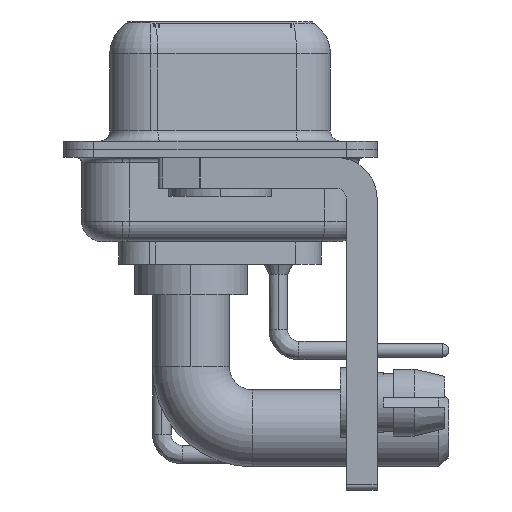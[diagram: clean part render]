
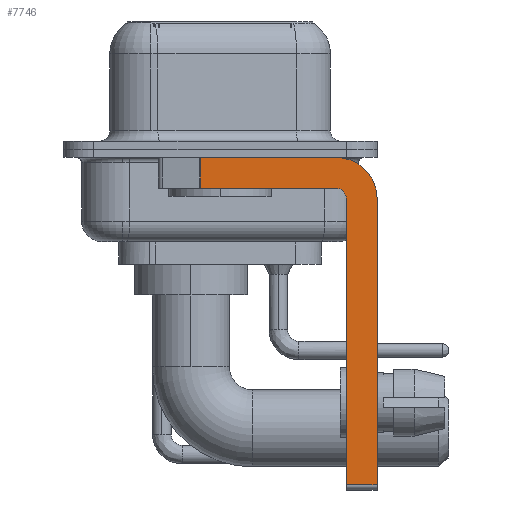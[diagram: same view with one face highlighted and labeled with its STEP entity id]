
A CAD part, left-side view. The second image highlights one B-rep face of the part: STEP entity #7746.
In plain terms, the highlighted planar face has unit normal (-1, 0, 0).
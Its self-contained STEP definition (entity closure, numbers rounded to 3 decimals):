
#274 = ORIENTED_EDGE ( 'NONE', *, *, #30336, .F. ) ;
#1246 = CARTESIAN_POINT ( 'NONE',  ( -2.9, -5.65, -16.35 ) ) ;
#1371 = AXIS2_PLACEMENT_3D ( 'NONE', #30924, #18235, #26679 ) ;
#1701 = CARTESIAN_POINT ( 'NONE',  ( -2.9, 0.978, -1.9 ) ) ;
#1873 = LINE ( 'NONE', #1701, #7406 ) ;
#1939 = DIRECTION ( 'NONE',  ( 0., 0., 1. ) ) ;
#2439 = EDGE_CURVE ( 'NONE', #2529, #18310, #12420, .T. ) ;
#2529 = VERTEX_POINT ( 'NONE', #21902 ) ;
#2671 = CIRCLE ( 'NONE', #26394, 2. ) ;
#3564 = CARTESIAN_POINT ( 'NONE',  ( -2.9, -5.65, -0.4 ) ) ;
#4434 = DIRECTION ( 'NONE',  ( -1., 0., 0. ) ) ;
#4453 = VERTEX_POINT ( 'NONE', #32727 ) ;
#5607 = VECTOR ( 'NONE', #20358, 1000. ) ;
#6105 = CARTESIAN_POINT ( 'NONE',  ( -2.9, 0.978, -1.9 ) ) ;
#6236 = CARTESIAN_POINT ( 'NONE',  ( -2.9, -6.15, -2.4 ) ) ;
#6277 = EDGE_CURVE ( 'NONE', #17366, #2529, #15496, .T. ) ;
#6924 = VERTEX_POINT ( 'NONE', #25383 ) ;
#7406 = VECTOR ( 'NONE', #31577, 1000. ) ;
#7596 = CARTESIAN_POINT ( 'NONE',  ( -2.9, -5.65, -1.9 ) ) ;
#7746 = ADVANCED_FACE ( 'NONE', ( #12054 ), #9388, .F. ) ;
#8556 = EDGE_CURVE ( 'NONE', #6924, #4453, #12273, .T. ) ;
#8972 = CARTESIAN_POINT ( 'NONE',  ( -2.9, -5.65, -2.4 ) ) ;
#9377 = VECTOR ( 'NONE', #17422, 1000. ) ;
#9388 = PLANE ( 'NONE',  #1371 ) ;
#10765 = LINE ( 'NONE', #19258, #32249 ) ;
#12054 = FACE_OUTER_BOUND ( 'NONE', #18963, .T. ) ;
#12273 = LINE ( 'NONE', #23012, #9377 ) ;
#12295 = LINE ( 'NONE', #22341, #13647 ) ;
#12420 = LINE ( 'NONE', #7596, #13348 ) ;
#13260 = DIRECTION ( 'NONE',  ( 0., -1., 0. ) ) ;
#13348 = VECTOR ( 'NONE', #23149, 1000. ) ;
#13647 = VECTOR ( 'NONE', #31171, 1000. ) ;
#15496 = CIRCLE ( 'NONE', #33496, 0.5 ) ;
#15599 = ORIENTED_EDGE ( 'NONE', *, *, #6277, .F. ) ;
#15678 = ORIENTED_EDGE ( 'NONE', *, *, #23368, .T. ) ;
#16032 = EDGE_CURVE ( 'NONE', #19768, #18310, #1873, .T. ) ;
#16034 = EDGE_CURVE ( 'NONE', #29309, #17366, #12295, .T. ) ;
#16940 = ORIENTED_EDGE ( 'NONE', *, *, #2439, .F. ) ;
#17304 = DIRECTION ( 'NONE',  ( 0., 0., -1. ) ) ;
#17366 = VERTEX_POINT ( 'NONE', #6236 ) ;
#17422 = DIRECTION ( 'NONE',  ( 0., 0., -1. ) ) ;
#18219 = ORIENTED_EDGE ( 'NONE', *, *, #16032, .T. ) ;
#18235 = DIRECTION ( 'NONE',  ( 1., 0., 0. ) ) ;
#18310 = VERTEX_POINT ( 'NONE', #6105 ) ;
#18963 = EDGE_LOOP ( 'NONE', ( #26443, #18219, #16940, #15599, #32008, #15678, #29187, #274 ) ) ;
#19258 = CARTESIAN_POINT ( 'NONE',  ( -2.9, 3., -0.4 ) ) ;
#19768 = VERTEX_POINT ( 'NONE', #28091 ) ;
#20358 = DIRECTION ( 'NONE',  ( 0., -1., 0. ) ) ;
#21723 = CARTESIAN_POINT ( 'NONE',  ( -2.9, -6.15, -16.35 ) ) ;
#21902 = CARTESIAN_POINT ( 'NONE',  ( -2.9, -5.65, -1.9 ) ) ;
#22201 = DIRECTION ( 'NONE',  ( 1., 0., 0. ) ) ;
#22341 = CARTESIAN_POINT ( 'NONE',  ( -2.9, -6.15, -16.6 ) ) ;
#23012 = CARTESIAN_POINT ( 'NONE',  ( -2.9, -7.65, -2.4 ) ) ;
#23149 = DIRECTION ( 'NONE',  ( 0., 1., 0. ) ) ;
#23304 = VERTEX_POINT ( 'NONE', #3564 ) ;
#23368 = EDGE_CURVE ( 'NONE', #29309, #4453, #33747, .T. ) ;
#25383 = CARTESIAN_POINT ( 'NONE',  ( -2.9, -7.65, -2.4 ) ) ;
#26229 = EDGE_CURVE ( 'NONE', #19768, #23304, #10765, .T. ) ;
#26394 = AXIS2_PLACEMENT_3D ( 'NONE', #8972, #22201, #17304 ) ;
#26443 = ORIENTED_EDGE ( 'NONE', *, *, #26229, .F. ) ;
#26679 = DIRECTION ( 'NONE',  ( 0., 0., -1. ) ) ;
#28091 = CARTESIAN_POINT ( 'NONE',  ( -2.9, 0.978, -0.4 ) ) ;
#29187 = ORIENTED_EDGE ( 'NONE', *, *, #8556, .F. ) ;
#29309 = VERTEX_POINT ( 'NONE', #21723 ) ;
#30336 = EDGE_CURVE ( 'NONE', #23304, #6924, #2671, .T. ) ;
#30924 = CARTESIAN_POINT ( 'NONE',  ( -2.9, -5.65, -2.4 ) ) ;
#31171 = DIRECTION ( 'NONE',  ( 0., 0., 1. ) ) ;
#31577 = DIRECTION ( 'NONE',  ( 0., 0., -1. ) ) ;
#32008 = ORIENTED_EDGE ( 'NONE', *, *, #16034, .F. ) ;
#32249 = VECTOR ( 'NONE', #13260, 1000. ) ;
#32727 = CARTESIAN_POINT ( 'NONE',  ( -2.9, -7.65, -16.35 ) ) ;
#33496 = AXIS2_PLACEMENT_3D ( 'NONE', #34098, #4434, #1939 ) ;
#33747 = LINE ( 'NONE', #1246, #5607 ) ;
#34098 = CARTESIAN_POINT ( 'NONE',  ( -2.9, -5.65, -2.4 ) ) ;
